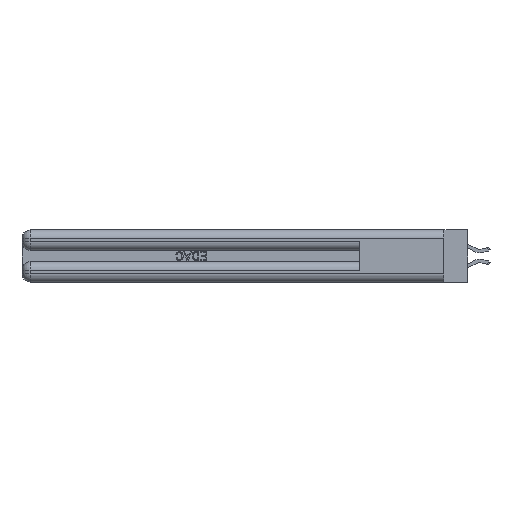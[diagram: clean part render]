
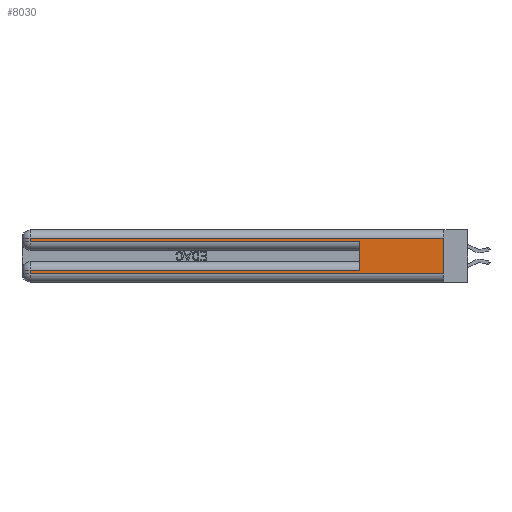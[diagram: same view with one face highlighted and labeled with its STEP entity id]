
A CAD part, left-side view. The second image highlights one B-rep face of the part: STEP entity #8030.
In plain terms, the highlighted planar face has unit normal (-1, 0, 0).
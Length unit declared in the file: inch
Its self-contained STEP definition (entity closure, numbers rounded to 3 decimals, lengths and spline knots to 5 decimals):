
#1001 = EDGE_CURVE ( 'NONE', #30914, #42773, #11705, .T. ) ;
#1669 = CARTESIAN_POINT ( 'NONE',  ( 0., 0., 0.285 ) ) ;
#1798 = LINE ( 'NONE', #27766, #11026 ) ;
#2084 = LINE ( 'NONE', #12308, #41272 ) ;
#2632 = CARTESIAN_POINT ( 'NONE',  ( 0., 0., 0.06 ) ) ;
#4491 = ORIENTED_EDGE ( 'NONE', *, *, #1001, .T. ) ;
#4723 = VECTOR ( 'NONE', #21024, 39.37008 ) ;
#5085 = DIRECTION ( 'NONE',  ( 0., 0., -1. ) ) ;
#5669 = CARTESIAN_POINT ( 'NONE',  ( 0., 2.94, 0.37 ) ) ;
#6807 = LINE ( 'NONE', #35878, #33489 ) ;
#7066 = DIRECTION ( 'NONE',  ( 0., 0., -1. ) ) ;
#7259 = DIRECTION ( 'NONE',  ( 0., -1., 0. ) ) ;
#7416 = LINE ( 'NONE', #2632, #22693 ) ;
#7902 = ORIENTED_EDGE ( 'NONE', *, *, #37027, .T. ) ;
#8030 = ADVANCED_FACE ( 'NONE', ( #34182 ), #12276, .F. ) ;
#8558 = ORIENTED_EDGE ( 'NONE', *, *, #34038, .T. ) ;
#9069 = EDGE_CURVE ( 'NONE', #41839, #30482, #7416, .T. ) ;
#10541 = CARTESIAN_POINT ( 'NONE',  ( 0., 0., 0.37 ) ) ;
#10614 = VECTOR ( 'NONE', #41610, 39.37008 ) ;
#11026 = VECTOR ( 'NONE', #20240, 39.37008 ) ;
#11029 = CARTESIAN_POINT ( 'NONE',  ( 0., 0., 0.06 ) ) ;
#11129 = EDGE_CURVE ( 'NONE', #19312, #32423, #1798, .T. ) ;
#11705 = LINE ( 'NONE', #17306, #10614 ) ;
#11819 = CARTESIAN_POINT ( 'NONE',  ( 0., 0.6, 0.085 ) ) ;
#12276 = PLANE ( 'NONE',  #14247 ) ;
#12308 = CARTESIAN_POINT ( 'NONE',  ( 0., 0.6, 0.145 ) ) ;
#14015 = CARTESIAN_POINT ( 'NONE',  ( 0., 0., 0.31 ) ) ;
#14063 = EDGE_CURVE ( 'NONE', #27319, #23768, #30422, .T. ) ;
#14247 = AXIS2_PLACEMENT_3D ( 'NONE', #15752, #18619, #5085 ) ;
#15418 = CARTESIAN_POINT ( 'NONE',  ( 0., 2.94, 0.06 ) ) ;
#15752 = CARTESIAN_POINT ( 'NONE',  ( 0., 0., 0.37 ) ) ;
#16744 = CARTESIAN_POINT ( 'NONE',  ( 0., 2.94, 0.085 ) ) ;
#17306 = CARTESIAN_POINT ( 'NONE',  ( 0., 0., 0.085 ) ) ;
#18619 = DIRECTION ( 'NONE',  ( 1., 0., 0. ) ) ;
#19312 = VERTEX_POINT ( 'NONE', #14015 ) ;
#19444 = DIRECTION ( 'NONE',  ( 0., 0., 1. ) ) ;
#20240 = DIRECTION ( 'NONE',  ( 0., 1., 0. ) ) ;
#20265 = CARTESIAN_POINT ( 'NONE',  ( 0., 2.94, 0.285 ) ) ;
#21024 = DIRECTION ( 'NONE',  ( 0., 0., -1. ) ) ;
#21850 = ORIENTED_EDGE ( 'NONE', *, *, #38784, .F. ) ;
#22693 = VECTOR ( 'NONE', #24790, 39.37008 ) ;
#23768 = VERTEX_POINT ( 'NONE', #24419 ) ;
#24266 = ORIENTED_EDGE ( 'NONE', *, *, #14063, .T. ) ;
#24419 = CARTESIAN_POINT ( 'NONE',  ( 0., 0.6, 0.285 ) ) ;
#24790 = DIRECTION ( 'NONE',  ( 0., -1., 0. ) ) ;
#24928 = VECTOR ( 'NONE', #7259, 39.37008 ) ;
#26866 = ORIENTED_EDGE ( 'NONE', *, *, #35240, .F. ) ;
#27319 = VERTEX_POINT ( 'NONE', #20265 ) ;
#27766 = CARTESIAN_POINT ( 'NONE',  ( 0., 0., 0.31 ) ) ;
#28091 = EDGE_LOOP ( 'NONE', ( #21850, #37693, #8558, #24266, #26866, #4491, #7902, #32925 ) ) ;
#30422 = LINE ( 'NONE', #1669, #24928 ) ;
#30482 = VERTEX_POINT ( 'NONE', #11029 ) ;
#30914 = VERTEX_POINT ( 'NONE', #11819 ) ;
#31551 = VECTOR ( 'NONE', #43836, 39.37008 ) ;
#31991 = CARTESIAN_POINT ( 'NONE',  ( 0., 2.94, 0.31 ) ) ;
#32423 = VERTEX_POINT ( 'NONE', #31991 ) ;
#32925 = ORIENTED_EDGE ( 'NONE', *, *, #9069, .T. ) ;
#33489 = VECTOR ( 'NONE', #7066, 39.37008 ) ;
#34038 = EDGE_CURVE ( 'NONE', #32423, #27319, #39739, .T. ) ;
#34182 = FACE_OUTER_BOUND ( 'NONE', #28091, .T. ) ;
#35240 = EDGE_CURVE ( 'NONE', #30914, #23768, #2084, .T. ) ;
#35878 = CARTESIAN_POINT ( 'NONE',  ( 0., 2.94, 0.37 ) ) ;
#37027 = EDGE_CURVE ( 'NONE', #42773, #41839, #6807, .T. ) ;
#37352 = LINE ( 'NONE', #10541, #4723 ) ;
#37693 = ORIENTED_EDGE ( 'NONE', *, *, #11129, .T. ) ;
#38784 = EDGE_CURVE ( 'NONE', #19312, #30482, #37352, .T. ) ;
#39739 = LINE ( 'NONE', #5669, #31551 ) ;
#41272 = VECTOR ( 'NONE', #19444, 39.37008 ) ;
#41610 = DIRECTION ( 'NONE',  ( 0., 1., 0. ) ) ;
#41839 = VERTEX_POINT ( 'NONE', #15418 ) ;
#42773 = VERTEX_POINT ( 'NONE', #16744 ) ;
#43836 = DIRECTION ( 'NONE',  ( 0., 0., -1. ) ) ;
